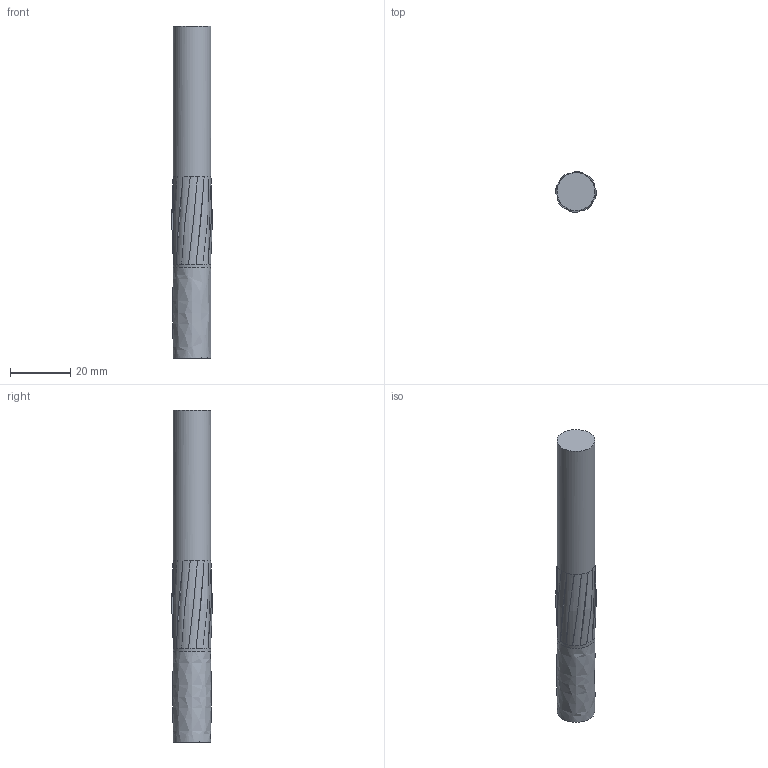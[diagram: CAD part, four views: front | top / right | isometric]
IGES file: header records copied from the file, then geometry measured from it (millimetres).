
Global section: file name: .50 bmg rifling button; native system: Autodesk Inventor 2017; preprocessor: unknown; author: user; date: 20201212.203015; units: millimetre
Bounding box: 13.52 x 13.52 x 110 mm (x, y, z)
Volume: 13831.6 mm3; surface area: 4805.1 mm2
Topology: 1 solids, 1 shells, 37 faces, 90 edges, 55 vertices
Faces by surface type: bspline 37
